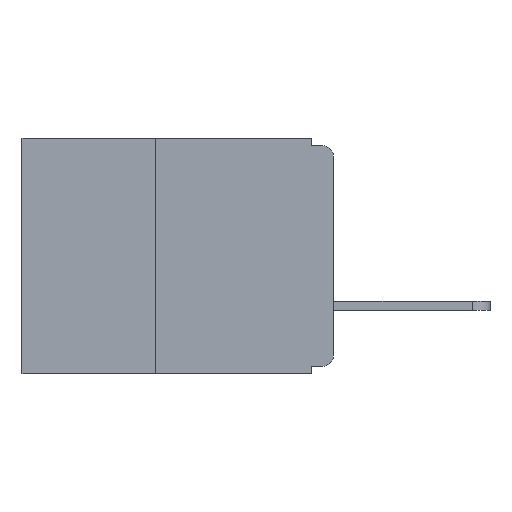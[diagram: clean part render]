
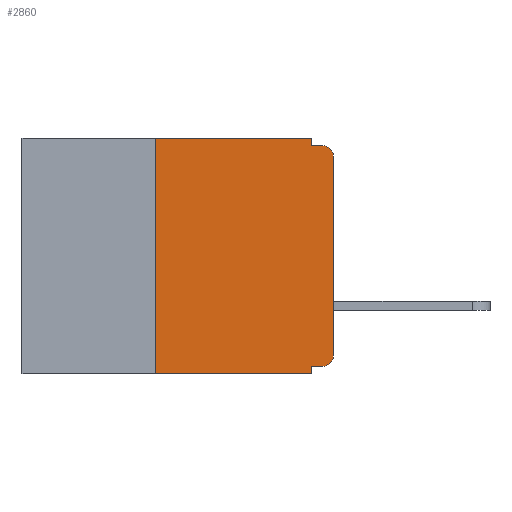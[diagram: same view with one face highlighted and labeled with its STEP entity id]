
A CAD part, left-side view. The second image highlights one B-rep face of the part: STEP entity #2860.
In plain terms, the highlighted planar face has unit normal (-1, 0, 0).
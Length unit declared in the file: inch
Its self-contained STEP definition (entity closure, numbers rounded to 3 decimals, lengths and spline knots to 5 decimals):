
#177 = VECTOR ( 'NONE', #13138, 39.37008 ) ;
#233 = DIRECTION ( 'NONE',  ( 0., 0., -1. ) ) ;
#263 = VECTOR ( 'NONE', #9614, 39.37008 ) ;
#292 = CARTESIAN_POINT ( 'NONE',  ( 0., 0.031, 0. ) ) ;
#295 = VERTEX_POINT ( 'NONE', #318 ) ;
#318 = CARTESIAN_POINT ( 'NONE',  ( 0., 0.031, -0.32 ) ) ;
#449 = EDGE_LOOP ( 'NONE', ( #11165, #7493, #14428, #11416, #9290, #4841, #514, #12133, #13260, #5117 ) ) ;
#514 = ORIENTED_EDGE ( 'NONE', *, *, #3260, .T. ) ;
#764 = AXIS2_PLACEMENT_3D ( 'NONE', #10691, #1788, #5361 ) ;
#832 = LINE ( 'NONE', #9769, #2855 ) ;
#901 = DIRECTION ( 'NONE',  ( 0., -1., 0. ) ) ;
#1544 = VECTOR ( 'NONE', #1994, 39.37008 ) ;
#1788 = DIRECTION ( 'NONE',  ( -1., 0., 0. ) ) ;
#1994 = DIRECTION ( 'NONE',  ( 0., 0., -1. ) ) ;
#2204 = CARTESIAN_POINT ( 'NONE',  ( 0., 0.015, -0.32 ) ) ;
#2382 = LINE ( 'NONE', #5042, #177 ) ;
#2415 = CIRCLE ( 'NONE', #764, 0.015 ) ;
#2521 = DIRECTION ( 'NONE',  ( 0., 0., -1. ) ) ;
#2852 = EDGE_CURVE ( 'NONE', #11863, #4673, #12390, .T. ) ;
#2855 = VECTOR ( 'NONE', #7445, 39.37008 ) ;
#2860 = ADVANCED_FACE ( 'NONE', ( #14931 ), #6632, .F. ) ;
#2988 = LINE ( 'NONE', #14926, #8378 ) ;
#3260 = EDGE_CURVE ( 'NONE', #13071, #14148, #2988, .T. ) ;
#3356 = LINE ( 'NONE', #9246, #3862 ) ;
#3430 = AXIS2_PLACEMENT_3D ( 'NONE', #4978, #7148, #2521 ) ;
#3862 = VECTOR ( 'NONE', #4485, 39.37008 ) ;
#3916 = EDGE_CURVE ( 'NONE', #6420, #295, #3356, .T. ) ;
#4136 = CARTESIAN_POINT ( 'NONE',  ( 0., 0.031, 0. ) ) ;
#4485 = DIRECTION ( 'NONE',  ( 0., 1., 0. ) ) ;
#4511 = CIRCLE ( 'NONE', #3430, 0.015 ) ;
#4550 = CARTESIAN_POINT ( 'NONE',  ( 0., 0.25, 0. ) ) ;
#4673 = VERTEX_POINT ( 'NONE', #7223 ) ;
#4782 = EDGE_CURVE ( 'NONE', #4673, #11355, #2415, .T. ) ;
#4841 = ORIENTED_EDGE ( 'NONE', *, *, #12487, .F. ) ;
#4976 = VECTOR ( 'NONE', #233, 39.37008 ) ;
#4978 = CARTESIAN_POINT ( 'NONE',  ( 0., 0.015, -0.305 ) ) ;
#5042 = CARTESIAN_POINT ( 'NONE',  ( 0., 0., -0.01 ) ) ;
#5092 = CARTESIAN_POINT ( 'NONE',  ( 0., 0.031, -0.33 ) ) ;
#5117 = ORIENTED_EDGE ( 'NONE', *, *, #6121, .T. ) ;
#5361 = DIRECTION ( 'NONE',  ( 0., 0., -1. ) ) ;
#5855 = EDGE_CURVE ( 'NONE', #8131, #11355, #2382, .T. ) ;
#6121 = EDGE_CURVE ( 'NONE', #6420, #11863, #4511, .T. ) ;
#6420 = VERTEX_POINT ( 'NONE', #2204 ) ;
#6597 = LINE ( 'NONE', #4136, #1544 ) ;
#6632 = PLANE ( 'NONE',  #13272 ) ;
#7148 = DIRECTION ( 'NONE',  ( -1., 0., 0. ) ) ;
#7223 = CARTESIAN_POINT ( 'NONE',  ( 0., 0., -0.025 ) ) ;
#7445 = DIRECTION ( 'NONE',  ( 0., 0., 1. ) ) ;
#7493 = ORIENTED_EDGE ( 'NONE', *, *, #4782, .T. ) ;
#7744 = DIRECTION ( 'NONE',  ( 0., 0., -1. ) ) ;
#7923 = LINE ( 'NONE', #13595, #9224 ) ;
#8038 = LINE ( 'NONE', #9884, #4976 ) ;
#8131 = VERTEX_POINT ( 'NONE', #13349 ) ;
#8378 = VECTOR ( 'NONE', #901, 39.37008 ) ;
#8494 = CARTESIAN_POINT ( 'NONE',  ( 0., 0., -0.305 ) ) ;
#8982 = DIRECTION ( 'NONE',  ( 1., 0., 0. ) ) ;
#9224 = VECTOR ( 'NONE', #9976, 39.37008 ) ;
#9246 = CARTESIAN_POINT ( 'NONE',  ( 0., 0., -0.32 ) ) ;
#9290 = ORIENTED_EDGE ( 'NONE', *, *, #10814, .F. ) ;
#9614 = DIRECTION ( 'NONE',  ( 0., 0., 1. ) ) ;
#9769 = CARTESIAN_POINT ( 'NONE',  ( 0., 0.25, -0.33 ) ) ;
#9884 = CARTESIAN_POINT ( 'NONE',  ( 0., 0.031, -0.33 ) ) ;
#9976 = DIRECTION ( 'NONE',  ( 0., -1., 0. ) ) ;
#10510 = VERTEX_POINT ( 'NONE', #4550 ) ;
#10691 = CARTESIAN_POINT ( 'NONE',  ( 0., 0.015, -0.025 ) ) ;
#10814 = EDGE_CURVE ( 'NONE', #10510, #11070, #7923, .T. ) ;
#11070 = VERTEX_POINT ( 'NONE', #292 ) ;
#11165 = ORIENTED_EDGE ( 'NONE', *, *, #2852, .T. ) ;
#11355 = VERTEX_POINT ( 'NONE', #14086 ) ;
#11416 = ORIENTED_EDGE ( 'NONE', *, *, #13124, .F. ) ;
#11863 = VERTEX_POINT ( 'NONE', #8494 ) ;
#12133 = ORIENTED_EDGE ( 'NONE', *, *, #13286, .F. ) ;
#12390 = LINE ( 'NONE', #12993, #263 ) ;
#12463 = CARTESIAN_POINT ( 'NONE',  ( 0., 0.437, 0. ) ) ;
#12487 = EDGE_CURVE ( 'NONE', #13071, #10510, #832, .T. ) ;
#12993 = CARTESIAN_POINT ( 'NONE',  ( 0., 0., 0. ) ) ;
#13071 = VERTEX_POINT ( 'NONE', #14466 ) ;
#13124 = EDGE_CURVE ( 'NONE', #11070, #8131, #6597, .T. ) ;
#13138 = DIRECTION ( 'NONE',  ( 0., -1., 0. ) ) ;
#13260 = ORIENTED_EDGE ( 'NONE', *, *, #3916, .F. ) ;
#13272 = AXIS2_PLACEMENT_3D ( 'NONE', #12463, #8982, #7744 ) ;
#13286 = EDGE_CURVE ( 'NONE', #295, #14148, #8038, .T. ) ;
#13349 = CARTESIAN_POINT ( 'NONE',  ( 0., 0.031, -0.01 ) ) ;
#13595 = CARTESIAN_POINT ( 'NONE',  ( 0., 0.437, 0. ) ) ;
#14086 = CARTESIAN_POINT ( 'NONE',  ( 0., 0.015, -0.01 ) ) ;
#14148 = VERTEX_POINT ( 'NONE', #5092 ) ;
#14428 = ORIENTED_EDGE ( 'NONE', *, *, #5855, .F. ) ;
#14466 = CARTESIAN_POINT ( 'NONE',  ( 0., 0.25, -0.33 ) ) ;
#14926 = CARTESIAN_POINT ( 'NONE',  ( 0., 0.437, -0.33 ) ) ;
#14931 = FACE_OUTER_BOUND ( 'NONE', #449, .T. ) ;
